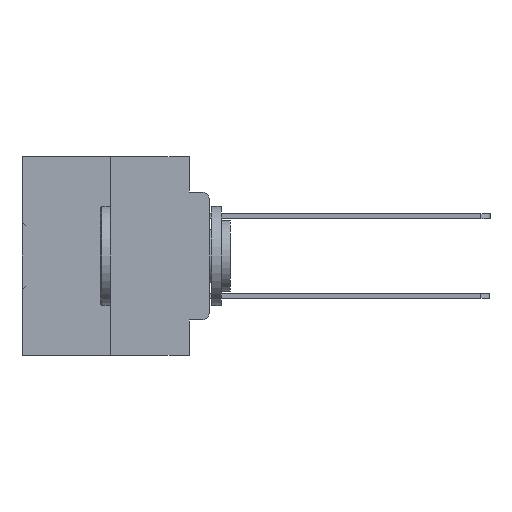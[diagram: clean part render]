
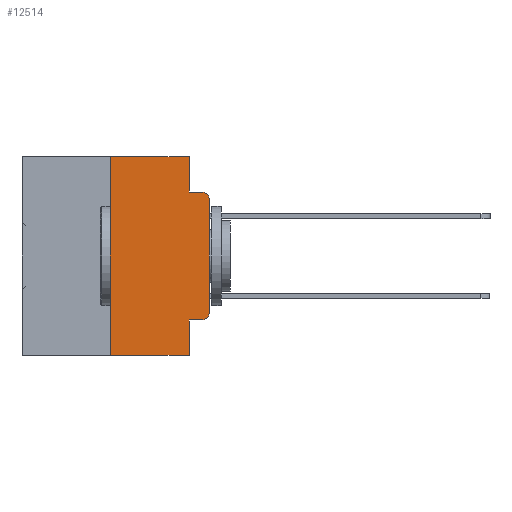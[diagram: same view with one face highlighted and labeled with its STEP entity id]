
A CAD part, left-side view. The second image highlights one B-rep face of the part: STEP entity #12514.
In plain terms, the highlighted planar face has unit normal (-1, 0, 0).
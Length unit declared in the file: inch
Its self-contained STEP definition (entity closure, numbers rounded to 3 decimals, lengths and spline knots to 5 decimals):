
#621 = EDGE_CURVE ( 'NONE', #20586, #15750, #26973, .T. ) ;
#702 = DIRECTION ( 'NONE',  ( -1., 0., 0. ) ) ;
#1203 = VECTOR ( 'NONE', #25151, 39.37008 ) ;
#1330 = EDGE_CURVE ( 'NONE', #33266, #28043, #26981, .T. ) ;
#2599 = FACE_OUTER_BOUND ( 'NONE', #27127, .T. ) ;
#2650 = VERTEX_POINT ( 'NONE', #19326 ) ;
#2925 = CARTESIAN_POINT ( 'NONE',  ( 0., 0.051, 0. ) ) ;
#2942 = CARTESIAN_POINT ( 'NONE',  ( 0., 0.02, -0.4115 ) ) ;
#3999 = EDGE_CURVE ( 'NONE', #22705, #28043, #14987, .T. ) ;
#4240 = DIRECTION ( 'NONE',  ( 0., 0., 1. ) ) ;
#5120 = EDGE_CURVE ( 'NONE', #22705, #8229, #28912, .T. ) ;
#5308 = CARTESIAN_POINT ( 'NONE',  ( 0., 0.473, 0. ) ) ;
#5555 = LINE ( 'NONE', #31833, #21249 ) ;
#5753 = DIRECTION ( 'NONE',  ( 0., 0., -1. ) ) ;
#6068 = VERTEX_POINT ( 'NONE', #30776 ) ;
#6311 = EDGE_CURVE ( 'NONE', #2650, #20586, #5555, .T. ) ;
#6716 = CARTESIAN_POINT ( 'NONE',  ( 0., 0.473, 0. ) ) ;
#6895 = DIRECTION ( 'NONE',  ( 0., 0., 1. ) ) ;
#7111 = AXIS2_PLACEMENT_3D ( 'NONE', #6716, #34172, #17988 ) ;
#7397 = ORIENTED_EDGE ( 'NONE', *, *, #3999, .T. ) ;
#7505 = VECTOR ( 'NONE', #35081, 39.37008 ) ;
#7733 = CARTESIAN_POINT ( 'NONE',  ( 0., 0.473, -0.5 ) ) ;
#7833 = ORIENTED_EDGE ( 'NONE', *, *, #621, .T. ) ;
#8229 = VERTEX_POINT ( 'NONE', #25197 ) ;
#9516 = AXIS2_PLACEMENT_3D ( 'NONE', #34686, #31282, #31200 ) ;
#11288 = CARTESIAN_POINT ( 'NONE',  ( 0., 0.02, -0.0885 ) ) ;
#11309 = VECTOR ( 'NONE', #5753, 39.37008 ) ;
#12201 = LINE ( 'NONE', #2925, #11309 ) ;
#12339 = DIRECTION ( 'NONE',  ( 0., -1., 0. ) ) ;
#12514 = ADVANCED_FACE ( 'NONE', ( #2599 ), #15219, .F. ) ;
#12855 = VERTEX_POINT ( 'NONE', #34066 ) ;
#13556 = AXIS2_PLACEMENT_3D ( 'NONE', #17545, #702, #20308 ) ;
#14272 = VECTOR ( 'NONE', #12339, 39.37008 ) ;
#14571 = EDGE_CURVE ( 'NONE', #12855, #6068, #12201, .T. ) ;
#14987 = LINE ( 'NONE', #7733, #7505 ) ;
#15219 = PLANE ( 'NONE',  #7111 ) ;
#15619 = CARTESIAN_POINT ( 'NONE',  ( 0., 0.051, 0. ) ) ;
#15750 = VERTEX_POINT ( 'NONE', #11288 ) ;
#15767 = ORIENTED_EDGE ( 'NONE', *, *, #1330, .F. ) ;
#16586 = DIRECTION ( 'NONE',  ( 0., -1., 0. ) ) ;
#17191 = DIRECTION ( 'NONE',  ( 0., 0., -1. ) ) ;
#17545 = CARTESIAN_POINT ( 'NONE',  ( 0., 0.02, -0.3915 ) ) ;
#17886 = CARTESIAN_POINT ( 'NONE',  ( 0., 0.25, -0.5 ) ) ;
#17988 = DIRECTION ( 'NONE',  ( 0., 0., -1. ) ) ;
#19326 = CARTESIAN_POINT ( 'NONE',  ( 0., 0., -0.3915 ) ) ;
#19636 = ORIENTED_EDGE ( 'NONE', *, *, #29340, .F. ) ;
#19712 = VERTEX_POINT ( 'NONE', #2942 ) ;
#19822 = LINE ( 'NONE', #5308, #26967 ) ;
#19834 = VECTOR ( 'NONE', #17191, 39.37008 ) ;
#20308 = DIRECTION ( 'NONE',  ( 0., 0., -1. ) ) ;
#20586 = VERTEX_POINT ( 'NONE', #31725 ) ;
#21249 = VECTOR ( 'NONE', #4240, 39.37008 ) ;
#21565 = CARTESIAN_POINT ( 'NONE',  ( 0., 0.051, -0.5 ) ) ;
#21714 = ORIENTED_EDGE ( 'NONE', *, *, #6311, .T. ) ;
#22435 = CARTESIAN_POINT ( 'NONE',  ( 0., 0.051, -0.4115 ) ) ;
#22705 = VERTEX_POINT ( 'NONE', #17886 ) ;
#23426 = LINE ( 'NONE', #22435, #1203 ) ;
#24365 = EDGE_CURVE ( 'NONE', #19712, #2650, #35272, .T. ) ;
#25098 = ORIENTED_EDGE ( 'NONE', *, *, #14571, .F. ) ;
#25151 = DIRECTION ( 'NONE',  ( 0., -1., 0. ) ) ;
#25197 = CARTESIAN_POINT ( 'NONE',  ( 0., 0.25, 0. ) ) ;
#26967 = VECTOR ( 'NONE', #16586, 39.37008 ) ;
#26973 = CIRCLE ( 'NONE', #9516, 0.02 ) ;
#26981 = LINE ( 'NONE', #15619, #19834 ) ;
#27127 = EDGE_LOOP ( 'NONE', ( #21714, #7833, #30613, #25098, #19636, #28480, #7397, #15767, #31910, #33572 ) ) ;
#28043 = VERTEX_POINT ( 'NONE', #21565 ) ;
#28480 = ORIENTED_EDGE ( 'NONE', *, *, #5120, .F. ) ;
#28648 = CARTESIAN_POINT ( 'NONE',  ( 0., 0.051, -0.0885 ) ) ;
#28744 = LINE ( 'NONE', #28648, #14272 ) ;
#28912 = LINE ( 'NONE', #34224, #35206 ) ;
#29340 = EDGE_CURVE ( 'NONE', #8229, #12855, #19822, .T. ) ;
#30613 = ORIENTED_EDGE ( 'NONE', *, *, #34549, .F. ) ;
#30776 = CARTESIAN_POINT ( 'NONE',  ( 0., 0.051, -0.0885 ) ) ;
#30992 = CARTESIAN_POINT ( 'NONE',  ( 0., 0.051, -0.4115 ) ) ;
#31200 = DIRECTION ( 'NONE',  ( 0., 0., -1. ) ) ;
#31282 = DIRECTION ( 'NONE',  ( -1., 0., 0. ) ) ;
#31660 = EDGE_CURVE ( 'NONE', #33266, #19712, #23426, .T. ) ;
#31725 = CARTESIAN_POINT ( 'NONE',  ( 0., 0., -0.1085 ) ) ;
#31833 = CARTESIAN_POINT ( 'NONE',  ( 0., 0., 0. ) ) ;
#31910 = ORIENTED_EDGE ( 'NONE', *, *, #31660, .T. ) ;
#33266 = VERTEX_POINT ( 'NONE', #30992 ) ;
#33572 = ORIENTED_EDGE ( 'NONE', *, *, #24365, .T. ) ;
#34066 = CARTESIAN_POINT ( 'NONE',  ( 0., 0.051, 0. ) ) ;
#34172 = DIRECTION ( 'NONE',  ( 1., 0., 0. ) ) ;
#34224 = CARTESIAN_POINT ( 'NONE',  ( 0., 0.25, 0. ) ) ;
#34549 = EDGE_CURVE ( 'NONE', #6068, #15750, #28744, .T. ) ;
#34686 = CARTESIAN_POINT ( 'NONE',  ( 0., 0.02, -0.1085 ) ) ;
#35081 = DIRECTION ( 'NONE',  ( 0., -1., 0. ) ) ;
#35206 = VECTOR ( 'NONE', #6895, 39.37008 ) ;
#35272 = CIRCLE ( 'NONE', #13556, 0.02 ) ;
